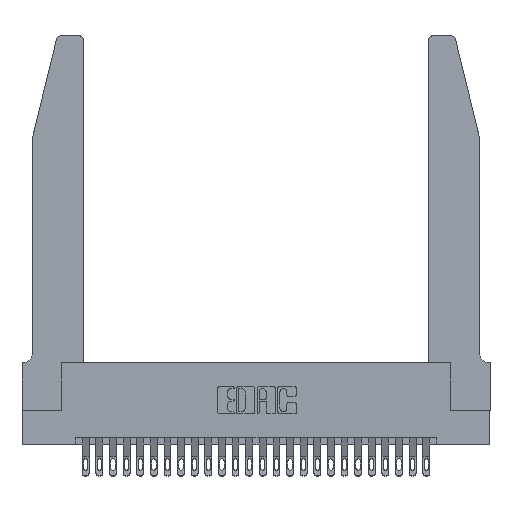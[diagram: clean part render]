
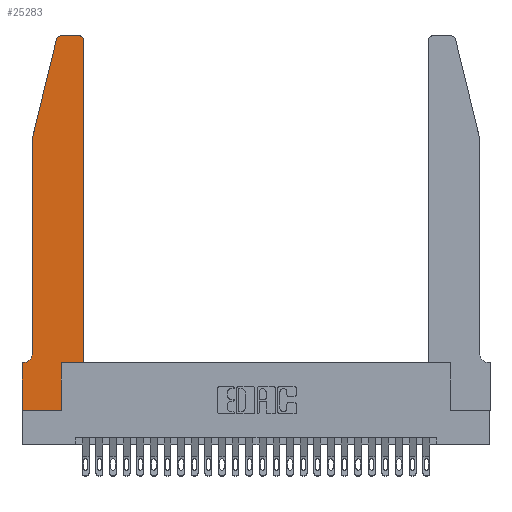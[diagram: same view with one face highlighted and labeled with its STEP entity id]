
A CAD part, top view. The second image highlights one B-rep face of the part: STEP entity #25283.
In plain terms, the highlighted planar face has unit normal (0, 0, 1).
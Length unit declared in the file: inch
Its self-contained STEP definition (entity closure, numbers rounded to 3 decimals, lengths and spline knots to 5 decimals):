
#108 = LINE ( 'NONE', #424, #10826 ) ;
#424 = CARTESIAN_POINT ( 'NONE',  ( 0.2865, 0.35, 0.37 ) ) ;
#875 = CARTESIAN_POINT ( 'NONE',  ( 0.4205, 2.75, 0.37 ) ) ;
#1260 = EDGE_CURVE ( 'NONE', #19471, #2585, #14251, .T. ) ;
#1336 = CARTESIAN_POINT ( 'NONE',  ( 0., 0., 0.37 ) ) ;
#1350 = VERTEX_POINT ( 'NONE', #16307 ) ;
#1371 = CARTESIAN_POINT ( 'NONE',  ( 0.284, 2.72, 0.37 ) ) ;
#1529 = DIRECTION ( 'NONE',  ( 0., 1., 0. ) ) ;
#1684 = VERTEX_POINT ( 'NONE', #26473 ) ;
#1881 = AXIS2_PLACEMENT_3D ( 'NONE', #21276, #8451, #23405 ) ;
#2000 = VECTOR ( 'NONE', #7984, 39.37008 ) ;
#2239 = ORIENTED_EDGE ( 'NONE', *, *, #15730, .T. ) ;
#2585 = VERTEX_POINT ( 'NONE', #10983 ) ;
#2724 = CARTESIAN_POINT ( 'NONE',  ( 0., 0., 0.37 ) ) ;
#2742 = LINE ( 'NONE', #13327, #24796 ) ;
#2760 = CARTESIAN_POINT ( 'NONE',  ( 0.4505, 2.72, 0.37 ) ) ;
#3077 = ORIENTED_EDGE ( 'NONE', *, *, #8969, .T. ) ;
#3172 = EDGE_CURVE ( 'NONE', #11698, #10954, #2742, .T. ) ;
#3181 = VERTEX_POINT ( 'NONE', #2724 ) ;
#3519 = DIRECTION ( 'NONE',  ( 1., 0., 0. ) ) ;
#3675 = PLANE ( 'NONE',  #23019 ) ;
#3760 = CARTESIAN_POINT ( 'NONE',  ( 0.2865, 0., 0.37 ) ) ;
#3911 = ORIENTED_EDGE ( 'NONE', *, *, #8590, .T. ) ;
#4030 = ORIENTED_EDGE ( 'NONE', *, *, #9180, .T. ) ;
#4035 = DIRECTION ( 'NONE',  ( 1., 0., 0. ) ) ;
#4827 = DIRECTION ( 'NONE',  ( -1., 0., 0. ) ) ;
#4852 = EDGE_CURVE ( 'NONE', #14214, #3181, #12741, .T. ) ;
#5265 = ORIENTED_EDGE ( 'NONE', *, *, #14151, .T. ) ;
#6239 = AXIS2_PLACEMENT_3D ( 'NONE', #21373, #8551, #23509 ) ;
#6689 = CARTESIAN_POINT ( 'NONE',  ( 0.0755, 2., 0.37 ) ) ;
#7199 = VERTEX_POINT ( 'NONE', #20878 ) ;
#7459 = ORIENTED_EDGE ( 'NONE', *, *, #11164, .T. ) ;
#7932 = EDGE_CURVE ( 'NONE', #15371, #11698, #14917, .T. ) ;
#7984 = DIRECTION ( 'NONE',  ( 0., -1., 0. ) ) ;
#8002 = CARTESIAN_POINT ( 'NONE',  ( 0., 0.35, 0.37 ) ) ;
#8103 = CARTESIAN_POINT ( 'NONE',  ( 0., 0.35, 0.37 ) ) ;
#8451 = DIRECTION ( 'NONE',  ( 0., 0., 1. ) ) ;
#8542 = VECTOR ( 'NONE', #4827, 39.37008 ) ;
#8551 = DIRECTION ( 'NONE',  ( 0., 0., -1. ) ) ;
#8590 = EDGE_CURVE ( 'NONE', #2585, #15371, #26533, .T. ) ;
#8969 = EDGE_CURVE ( 'NONE', #27179, #1350, #108, .T. ) ;
#9180 = EDGE_CURVE ( 'NONE', #1350, #1684, #11840, .T. ) ;
#9723 = LINE ( 'NONE', #11106, #21123 ) ;
#9903 = CARTESIAN_POINT ( 'NONE',  ( 0.25487, 2.72718, 0.37 ) ) ;
#10140 = DIRECTION ( 'NONE',  ( 1., 0., 0. ) ) ;
#10824 = VERTEX_POINT ( 'NONE', #2760 ) ;
#10826 = VECTOR ( 'NONE', #19740, 39.37008 ) ;
#10954 = VERTEX_POINT ( 'NONE', #14006 ) ;
#10983 = CARTESIAN_POINT ( 'NONE',  ( 0.284, 2.75, 0.37 ) ) ;
#11106 = CARTESIAN_POINT ( 'NONE',  ( 0.0755, 0.35, 0.37 ) ) ;
#11164 = EDGE_CURVE ( 'NONE', #3181, #27179, #11668, .T. ) ;
#11647 = ORIENTED_EDGE ( 'NONE', *, *, #7932, .T. ) ;
#11668 = LINE ( 'NONE', #1336, #16668 ) ;
#11698 = VERTEX_POINT ( 'NONE', #24301 ) ;
#11840 = LINE ( 'NONE', #12577, #22564 ) ;
#12577 = CARTESIAN_POINT ( 'NONE',  ( 0.4505, 0.35, 0.37 ) ) ;
#12741 = LINE ( 'NONE', #22959, #2000 ) ;
#12979 = ORIENTED_EDGE ( 'NONE', *, *, #4852, .T. ) ;
#13206 = EDGE_CURVE ( 'NONE', #10824, #19471, #15901, .T. ) ;
#13327 = CARTESIAN_POINT ( 'NONE',  ( 0.0755, 2., 0.37 ) ) ;
#13852 = ORIENTED_EDGE ( 'NONE', *, *, #13206, .T. ) ;
#14006 = CARTESIAN_POINT ( 'NONE',  ( 0.0755, 0.42, 0.37 ) ) ;
#14151 = EDGE_CURVE ( 'NONE', #1684, #10824, #20883, .T. ) ;
#14214 = VERTEX_POINT ( 'NONE', #8103 ) ;
#14251 = LINE ( 'NONE', #20746, #8542 ) ;
#14917 = LINE ( 'NONE', #6689, #15594 ) ;
#15115 = AXIS2_PLACEMENT_3D ( 'NONE', #1371, #16356, #3519 ) ;
#15371 = VERTEX_POINT ( 'NONE', #9903 ) ;
#15594 = VECTOR ( 'NONE', #19547, 39.37008 ) ;
#15730 = EDGE_CURVE ( 'NONE', #7199, #14214, #9723, .T. ) ;
#15901 = CIRCLE ( 'NONE', #1881, 0.03 ) ;
#16307 = CARTESIAN_POINT ( 'NONE',  ( 0.2865, 0.35, 0.37 ) ) ;
#16356 = DIRECTION ( 'NONE',  ( 0., 0., 1. ) ) ;
#16668 = VECTOR ( 'NONE', #18483, 39.37008 ) ;
#18483 = DIRECTION ( 'NONE',  ( 1., 0., 0. ) ) ;
#18673 = CARTESIAN_POINT ( 'NONE',  ( 0.4505, 0.35, 0.37 ) ) ;
#19471 = VERTEX_POINT ( 'NONE', #875 ) ;
#19547 = DIRECTION ( 'NONE',  ( -0.239, -0.971, 0. ) ) ;
#19655 = ORIENTED_EDGE ( 'NONE', *, *, #3172, .T. ) ;
#19740 = DIRECTION ( 'NONE',  ( 0., 1., 0. ) ) ;
#20229 = VECTOR ( 'NONE', #1529, 39.37008 ) ;
#20334 = EDGE_CURVE ( 'NONE', #10954, #7199, #23816, .T. ) ;
#20746 = CARTESIAN_POINT ( 'NONE',  ( 0.2605, 2.75, 0.37 ) ) ;
#20878 = CARTESIAN_POINT ( 'NONE',  ( 0.0055, 0.35, 0.37 ) ) ;
#20883 = LINE ( 'NONE', #18673, #20229 ) ;
#21123 = VECTOR ( 'NONE', #23901, 39.37008 ) ;
#21276 = CARTESIAN_POINT ( 'NONE',  ( 0.4205, 2.72, 0.37 ) ) ;
#21373 = CARTESIAN_POINT ( 'NONE',  ( 0.0055, 0.42, 0.37 ) ) ;
#21840 = DIRECTION ( 'NONE',  ( 0., -1., 0. ) ) ;
#22564 = VECTOR ( 'NONE', #4035, 39.37008 ) ;
#22959 = CARTESIAN_POINT ( 'NONE',  ( 0., 0., 0.37 ) ) ;
#22976 = DIRECTION ( 'NONE',  ( 0., 0., 1. ) ) ;
#23019 = AXIS2_PLACEMENT_3D ( 'NONE', #8002, #22976, #10140 ) ;
#23059 = EDGE_LOOP ( 'NONE', ( #24438, #3911, #11647, #19655, #26077, #2239, #12979, #7459, #3077, #4030, #5265, #13852 ) ) ;
#23405 = DIRECTION ( 'NONE',  ( 1., 0., 0. ) ) ;
#23509 = DIRECTION ( 'NONE',  ( -1., 0., 0. ) ) ;
#23816 = CIRCLE ( 'NONE', #6239, 0.07 ) ;
#23901 = DIRECTION ( 'NONE',  ( -1., 0., 0. ) ) ;
#24301 = CARTESIAN_POINT ( 'NONE',  ( 0.0755, 2., 0.37 ) ) ;
#24438 = ORIENTED_EDGE ( 'NONE', *, *, #1260, .T. ) ;
#24796 = VECTOR ( 'NONE', #21840, 39.37008 ) ;
#25283 = ADVANCED_FACE ( 'NONE', ( #26662 ), #3675, .T. ) ;
#26077 = ORIENTED_EDGE ( 'NONE', *, *, #20334, .T. ) ;
#26473 = CARTESIAN_POINT ( 'NONE',  ( 0.4505, 0.35, 0.37 ) ) ;
#26533 = CIRCLE ( 'NONE', #15115, 0.03 ) ;
#26662 = FACE_OUTER_BOUND ( 'NONE', #23059, .T. ) ;
#27179 = VERTEX_POINT ( 'NONE', #3760 ) ;
